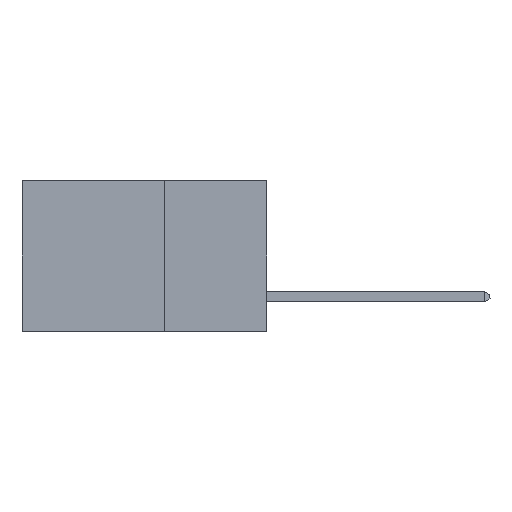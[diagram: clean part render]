
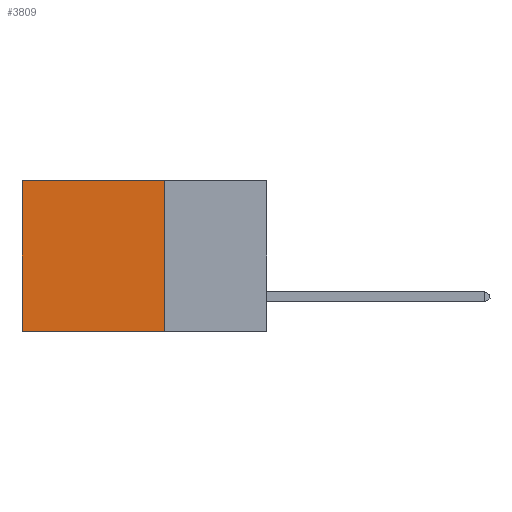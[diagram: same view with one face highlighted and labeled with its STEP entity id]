
A CAD part, left-side view. The second image highlights one B-rep face of the part: STEP entity #3809.
In plain terms, the highlighted planar face has unit normal (-1, 0, 0).
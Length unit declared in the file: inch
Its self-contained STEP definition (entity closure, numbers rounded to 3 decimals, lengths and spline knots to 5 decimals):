
#535 = VECTOR ( 'NONE', #1158, 39.37008 ) ;
#694 = CARTESIAN_POINT ( 'NONE',  ( 0.2875, 0.25, 0. ) ) ;
#1158 = DIRECTION ( 'NONE',  ( 0., 0., -1. ) ) ;
#2452 = FACE_OUTER_BOUND ( 'NONE', #15126, .T. ) ;
#2597 = VERTEX_POINT ( 'NONE', #14522 ) ;
#3809 = ADVANCED_FACE ( 'NONE', ( #2452 ), #13931, .F. ) ;
#5684 = EDGE_CURVE ( 'NONE', #2597, #11717, #20078, .T. ) ;
#5865 = DIRECTION ( 'NONE',  ( 0., 1., 0. ) ) ;
#6389 = LINE ( 'NONE', #694, #37419 ) ;
#6731 = VERTEX_POINT ( 'NONE', #20256 ) ;
#7759 = AXIS2_PLACEMENT_3D ( 'NONE', #34991, #38002, #20018 ) ;
#9578 = LINE ( 'NONE', #16152, #535 ) ;
#10075 = CARTESIAN_POINT ( 'NONE',  ( 0.2875, 0.25, -0.37 ) ) ;
#11717 = VERTEX_POINT ( 'NONE', #18406 ) ;
#13678 = EDGE_CURVE ( 'NONE', #25936, #6731, #23065, .T. ) ;
#13931 = PLANE ( 'NONE',  #7759 ) ;
#14106 = CARTESIAN_POINT ( 'NONE',  ( 0.2875, 0.25, -0.37 ) ) ;
#14522 = CARTESIAN_POINT ( 'NONE',  ( 0.2875, 0.25, 0. ) ) ;
#15126 = EDGE_LOOP ( 'NONE', ( #33852, #21543, #27712, #33191 ) ) ;
#16152 = CARTESIAN_POINT ( 'NONE',  ( 0.2875, 0.6, 0. ) ) ;
#18406 = CARTESIAN_POINT ( 'NONE',  ( 0.2875, 0.6, 0. ) ) ;
#20018 = DIRECTION ( 'NONE',  ( 0., 0., -1. ) ) ;
#20078 = LINE ( 'NONE', #20839, #34170 ) ;
#20256 = CARTESIAN_POINT ( 'NONE',  ( 0.2875, 0.6, -0.37 ) ) ;
#20839 = CARTESIAN_POINT ( 'NONE',  ( 0.2875, 0.25, 0. ) ) ;
#21543 = ORIENTED_EDGE ( 'NONE', *, *, #13678, .F. ) ;
#21793 = DIRECTION ( 'NONE',  ( 0., 0., -1. ) ) ;
#23065 = LINE ( 'NONE', #10075, #31083 ) ;
#25936 = VERTEX_POINT ( 'NONE', #14106 ) ;
#27712 = ORIENTED_EDGE ( 'NONE', *, *, #29500, .F. ) ;
#29500 = EDGE_CURVE ( 'NONE', #2597, #25936, #6389, .T. ) ;
#30895 = EDGE_CURVE ( 'NONE', #11717, #6731, #9578, .T. ) ;
#31083 = VECTOR ( 'NONE', #34112, 39.37008 ) ;
#33191 = ORIENTED_EDGE ( 'NONE', *, *, #5684, .T. ) ;
#33852 = ORIENTED_EDGE ( 'NONE', *, *, #30895, .T. ) ;
#34112 = DIRECTION ( 'NONE',  ( 0., 1., 0. ) ) ;
#34170 = VECTOR ( 'NONE', #5865, 39.37008 ) ;
#34991 = CARTESIAN_POINT ( 'NONE',  ( 0.2875, 0.25, 0. ) ) ;
#37419 = VECTOR ( 'NONE', #21793, 39.37008 ) ;
#38002 = DIRECTION ( 'NONE',  ( 1., 0., 0. ) ) ;
